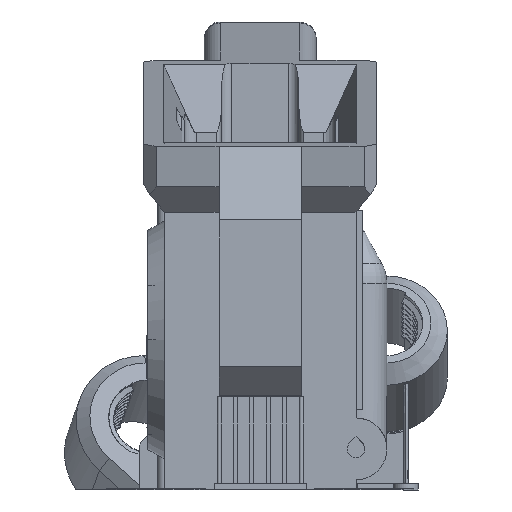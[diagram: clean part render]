
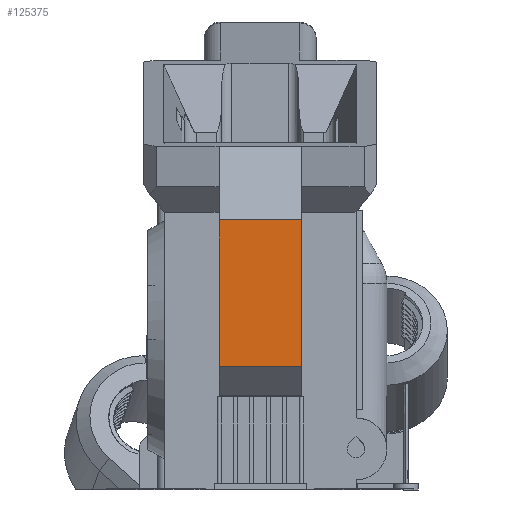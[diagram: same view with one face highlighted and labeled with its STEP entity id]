
A CAD part, left-side view. The second image highlights one B-rep face of the part: STEP entity #125375.
In plain terms, the highlighted planar face has unit normal (-1, 0, 0).
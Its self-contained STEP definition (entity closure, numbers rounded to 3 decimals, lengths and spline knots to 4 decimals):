
#3199 = LINE ( 'NONE', #109179, #16814 ) ;
#8737 = CARTESIAN_POINT ( 'NONE',  ( -4.237, 0.6526, 2.4712 ) ) ;
#11550 = LINE ( 'NONE', #37261, #106441 ) ;
#16814 = VECTOR ( 'NONE', #139991, 39.3701 ) ;
#19183 = AXIS2_PLACEMENT_3D ( 'NONE', #69707, #70324, #99324 ) ;
#29259 = CARTESIAN_POINT ( 'NONE',  ( -4.237, 0.6526, 1.5282 ) ) ;
#37261 = CARTESIAN_POINT ( 'NONE',  ( -4.237, 2.4558, 2.4712 ) ) ;
#46679 = CARTESIAN_POINT ( 'NONE',  ( -4.237, 1.1526, 1.5782 ) ) ;
#60126 = CARTESIAN_POINT ( 'NONE',  ( -4.237, 2.4558, 1.5782 ) ) ;
#64352 = ORIENTED_EDGE ( 'NONE', *, *, #114645, .F. ) ;
#69707 = CARTESIAN_POINT ( 'NONE',  ( -4.237, 2.4558, 1.5282 ) ) ;
#69767 = EDGE_CURVE ( 'NONE', #135652, #164280, #182430, .T. ) ;
#70324 = DIRECTION ( 'NONE',  ( -1., 0., 0. ) ) ;
#99324 = DIRECTION ( 'NONE',  ( 0., 0., 1. ) ) ;
#105789 = EDGE_CURVE ( 'NONE', #144269, #144798, #3199, .T. ) ;
#106441 = VECTOR ( 'NONE', #138531, 39.3701 ) ;
#107388 = ORIENTED_EDGE ( 'NONE', *, *, #105789, .F. ) ;
#108057 = VECTOR ( 'NONE', #128299, 39.3701 ) ;
#109179 = CARTESIAN_POINT ( 'NONE',  ( -4.237, 1.1526, 1.5282 ) ) ;
#114645 = EDGE_CURVE ( 'NONE', #144798, #135652, #11550, .T. ) ;
#119271 = EDGE_LOOP ( 'NONE', ( #127923, #176741, #64352, #107388 ) ) ;
#125375 = ADVANCED_FACE ( 'NONE', ( #140468 ), #156714, .T. ) ;
#127923 = ORIENTED_EDGE ( 'NONE', *, *, #129303, .F. ) ;
#128299 = DIRECTION ( 'NONE',  ( 0., 0., -1. ) ) ;
#129303 = EDGE_CURVE ( 'NONE', #164280, #144269, #133848, .T. ) ;
#133848 = LINE ( 'NONE', #60126, #142866 ) ;
#135652 = VERTEX_POINT ( 'NONE', #8737 ) ;
#138531 = DIRECTION ( 'NONE',  ( 0., -1., 0. ) ) ;
#139991 = DIRECTION ( 'NONE',  ( 0., 0., 1. ) ) ;
#140468 = FACE_OUTER_BOUND ( 'NONE', #119271, .T. ) ;
#142866 = VECTOR ( 'NONE', #149019, 39.3701 ) ;
#144269 = VERTEX_POINT ( 'NONE', #46679 ) ;
#144798 = VERTEX_POINT ( 'NONE', #172689 ) ;
#149019 = DIRECTION ( 'NONE',  ( 0., 1., 0. ) ) ;
#156714 = PLANE ( 'NONE',  #19183 ) ;
#164280 = VERTEX_POINT ( 'NONE', #177437 ) ;
#172689 = CARTESIAN_POINT ( 'NONE',  ( -4.237, 1.1526, 2.4712 ) ) ;
#176741 = ORIENTED_EDGE ( 'NONE', *, *, #69767, .F. ) ;
#177437 = CARTESIAN_POINT ( 'NONE',  ( -4.237, 0.6526, 1.5782 ) ) ;
#182430 = LINE ( 'NONE', #29259, #108057 ) ;
